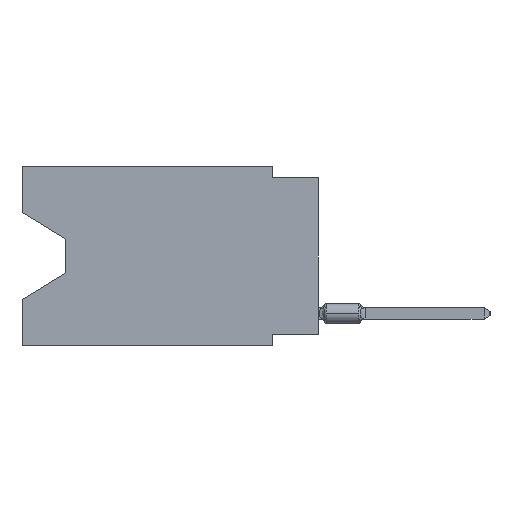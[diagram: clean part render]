
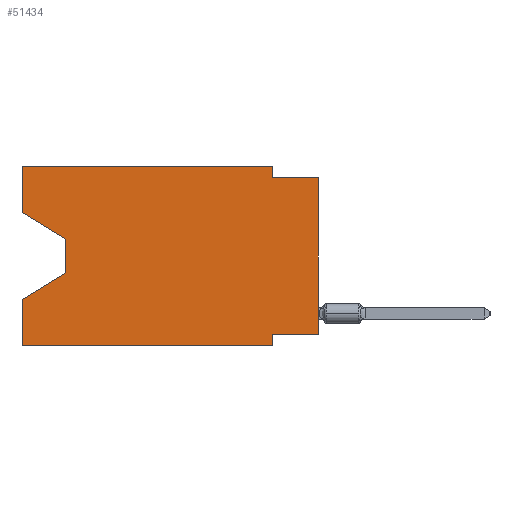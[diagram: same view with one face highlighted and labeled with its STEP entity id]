
A CAD part, left-side view. The second image highlights one B-rep face of the part: STEP entity #51434.
In plain terms, the highlighted planar face has unit normal (-1, 0, 0).
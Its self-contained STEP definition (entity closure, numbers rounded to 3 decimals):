
#2523 = EDGE_CURVE ( 'NONE', #49905, #30091, #36290, .T. ) ;
#2689 = CARTESIAN_POINT ( 'NONE',  ( 0., 16.383, 0. ) ) ;
#3319 = VERTEX_POINT ( 'NONE', #22929 ) ;
#3392 = LINE ( 'NONE', #83688, #60274 ) ;
#3678 = CARTESIAN_POINT ( 'NONE',  ( 0., 13.97, -5.893 ) ) ;
#4700 = ORIENTED_EDGE ( 'NONE', *, *, #15615, .F. ) ;
#6772 = VECTOR ( 'NONE', #25361, 1000. ) ;
#7742 = DIRECTION ( 'NONE',  ( 0., 0., -1. ) ) ;
#9974 = VECTOR ( 'NONE', #84638, 1000. ) ;
#12750 = CARTESIAN_POINT ( 'NONE',  ( 0., 0., -0.635 ) ) ;
#13230 = CARTESIAN_POINT ( 'NONE',  ( 0., 0., -9.271 ) ) ;
#13861 = VECTOR ( 'NONE', #78822, 1000. ) ;
#13897 = EDGE_CURVE ( 'NONE', #53488, #20159, #19258, .T. ) ;
#14286 = VECTOR ( 'NONE', #51158, 1000. ) ;
#14337 = VERTEX_POINT ( 'NONE', #32189 ) ;
#15088 = VECTOR ( 'NONE', #86462, 1000. ) ;
#15160 = DIRECTION ( 'NONE',  ( 0., 0., -1. ) ) ;
#15384 = VERTEX_POINT ( 'NONE', #83259 ) ;
#15615 = EDGE_CURVE ( 'NONE', #30091, #77442, #48062, .T. ) ;
#17191 = ORIENTED_EDGE ( 'NONE', *, *, #45602, .F. ) ;
#17448 = VECTOR ( 'NONE', #7742, 1000. ) ;
#17941 = CARTESIAN_POINT ( 'NONE',  ( 0., 16.383, 0. ) ) ;
#18645 = VECTOR ( 'NONE', #30458, 1000. ) ;
#19130 = DIRECTION ( 'NONE',  ( 1., 0., 0. ) ) ;
#19258 = LINE ( 'NONE', #17941, #9974 ) ;
#20159 = VERTEX_POINT ( 'NONE', #23409 ) ;
#21346 = VERTEX_POINT ( 'NONE', #3678 ) ;
#22929 = CARTESIAN_POINT ( 'NONE',  ( 0., 2.54, -0.635 ) ) ;
#23409 = CARTESIAN_POINT ( 'NONE',  ( 0., 16.383, 0. ) ) ;
#23968 = VECTOR ( 'NONE', #47312, 1000. ) ;
#25361 = DIRECTION ( 'NONE',  ( 0., -1., 0. ) ) ;
#26117 = EDGE_CURVE ( 'NONE', #21346, #15384, #30984, .T. ) ;
#26869 = ORIENTED_EDGE ( 'NONE', *, *, #61864, .F. ) ;
#27092 = EDGE_CURVE ( 'NONE', #14337, #77442, #79808, .T. ) ;
#27497 = VECTOR ( 'NONE', #15160, 1000. ) ;
#29327 = CARTESIAN_POINT ( 'NONE',  ( 0., 2.54, 0. ) ) ;
#29584 = CARTESIAN_POINT ( 'NONE',  ( 0., 0., -0.635 ) ) ;
#30091 = VERTEX_POINT ( 'NONE', #38604 ) ;
#30117 = LINE ( 'NONE', #83649, #14286 ) ;
#30458 = DIRECTION ( 'NONE',  ( 0., 0., 1. ) ) ;
#30984 = LINE ( 'NONE', #77511, #13861 ) ;
#32189 = CARTESIAN_POINT ( 'NONE',  ( 0., 16.383, -9.906 ) ) ;
#33269 = CARTESIAN_POINT ( 'NONE',  ( 0., 13.97, -4.013 ) ) ;
#34219 = LINE ( 'NONE', #67194, #76534 ) ;
#34500 = ORIENTED_EDGE ( 'NONE', *, *, #13897, .F. ) ;
#34548 = EDGE_CURVE ( 'NONE', #58864, #21346, #34219, .T. ) ;
#36290 = LINE ( 'NONE', #43300, #57876 ) ;
#38604 = CARTESIAN_POINT ( 'NONE',  ( 0., 2.54, -9.271 ) ) ;
#39516 = DIRECTION ( 'NONE',  ( 0., 0., -1. ) ) ;
#43300 = CARTESIAN_POINT ( 'NONE',  ( 0., 0., -9.271 ) ) ;
#43328 = EDGE_LOOP ( 'NONE', ( #52290, #75927, #78008, #64003, #60770, #4700, #72582, #62043, #17191, #57909, #26869, #34500 ) ) ;
#43611 = CARTESIAN_POINT ( 'NONE',  ( 0., 2.54, 0. ) ) ;
#45602 = EDGE_CURVE ( 'NONE', #3319, #58259, #75779, .T. ) ;
#47312 = DIRECTION ( 'NONE',  ( 0., -1., 0. ) ) ;
#47644 = CARTESIAN_POINT ( 'NONE',  ( 0., 2.54, -9.906 ) ) ;
#48062 = LINE ( 'NONE', #47644, #17448 ) ;
#48789 = CARTESIAN_POINT ( 'NONE',  ( 0., 16.383, -2.546 ) ) ;
#49905 = VERTEX_POINT ( 'NONE', #13230 ) ;
#50199 = CARTESIAN_POINT ( 'NONE',  ( 0., 0., 0. ) ) ;
#50317 = DIRECTION ( 'NONE',  ( 0., 0., 1. ) ) ;
#50628 = LINE ( 'NONE', #50199, #18645 ) ;
#50756 = DIRECTION ( 'NONE',  ( 0., 1., 0. ) ) ;
#50798 = CARTESIAN_POINT ( 'NONE',  ( 0., 2.54, -9.906 ) ) ;
#51158 = DIRECTION ( 'NONE',  ( 0., -0.855, -0.519 ) ) ;
#51351 = EDGE_CURVE ( 'NONE', #53488, #58864, #30117, .T. ) ;
#51434 = ADVANCED_FACE ( 'NONE', ( #86247 ), #79253, .F. ) ;
#52290 = ORIENTED_EDGE ( 'NONE', *, *, #51351, .T. ) ;
#53488 = VERTEX_POINT ( 'NONE', #48789 ) ;
#54642 = EDGE_CURVE ( 'NONE', #49905, #58259, #50628, .T. ) ;
#57876 = VECTOR ( 'NONE', #50756, 1000. ) ;
#57909 = ORIENTED_EDGE ( 'NONE', *, *, #59511, .F. ) ;
#58259 = VERTEX_POINT ( 'NONE', #29584 ) ;
#58864 = VERTEX_POINT ( 'NONE', #33269 ) ;
#59501 = DIRECTION ( 'NONE',  ( 0., 0., -1. ) ) ;
#59511 = EDGE_CURVE ( 'NONE', #77238, #3319, #69971, .T. ) ;
#60274 = VECTOR ( 'NONE', #50317, 1000. ) ;
#60770 = ORIENTED_EDGE ( 'NONE', *, *, #27092, .T. ) ;
#61864 = EDGE_CURVE ( 'NONE', #20159, #77238, #78892, .T. ) ;
#62043 = ORIENTED_EDGE ( 'NONE', *, *, #54642, .T. ) ;
#64003 = ORIENTED_EDGE ( 'NONE', *, *, #75261, .F. ) ;
#67194 = CARTESIAN_POINT ( 'NONE',  ( 0., 13.97, -4.013 ) ) ;
#69971 = LINE ( 'NONE', #43611, #27497 ) ;
#72582 = ORIENTED_EDGE ( 'NONE', *, *, #2523, .F. ) ;
#75261 = EDGE_CURVE ( 'NONE', #14337, #15384, #3392, .T. ) ;
#75779 = LINE ( 'NONE', #12750, #15088 ) ;
#75913 = AXIS2_PLACEMENT_3D ( 'NONE', #80114, #19130, #59501 ) ;
#75927 = ORIENTED_EDGE ( 'NONE', *, *, #34548, .T. ) ;
#76534 = VECTOR ( 'NONE', #39516, 1000. ) ;
#77238 = VERTEX_POINT ( 'NONE', #29327 ) ;
#77442 = VERTEX_POINT ( 'NONE', #50798 ) ;
#77511 = CARTESIAN_POINT ( 'NONE',  ( 0., 13.97, -5.893 ) ) ;
#78008 = ORIENTED_EDGE ( 'NONE', *, *, #26117, .T. ) ;
#78822 = DIRECTION ( 'NONE',  ( 0., 0.855, -0.519 ) ) ;
#78892 = LINE ( 'NONE', #2689, #6772 ) ;
#79253 = PLANE ( 'NONE',  #75913 ) ;
#79808 = LINE ( 'NONE', #80245, #23968 ) ;
#80114 = CARTESIAN_POINT ( 'NONE',  ( 0., 16.383, 0. ) ) ;
#80245 = CARTESIAN_POINT ( 'NONE',  ( 0., 16.383, -9.906 ) ) ;
#83259 = CARTESIAN_POINT ( 'NONE',  ( 0., 16.383, -7.36 ) ) ;
#83649 = CARTESIAN_POINT ( 'NONE',  ( 0., 16.383, -2.546 ) ) ;
#83688 = CARTESIAN_POINT ( 'NONE',  ( 0., 16.383, 0. ) ) ;
#84638 = DIRECTION ( 'NONE',  ( 0., 0., 1. ) ) ;
#86247 = FACE_OUTER_BOUND ( 'NONE', #43328, .T. ) ;
#86462 = DIRECTION ( 'NONE',  ( 0., -1., 0. ) ) ;
